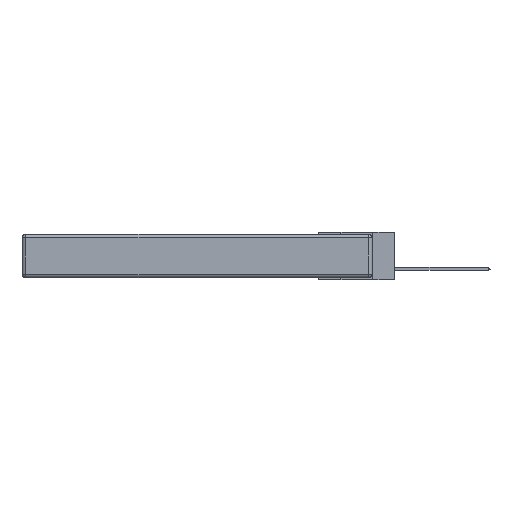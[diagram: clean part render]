
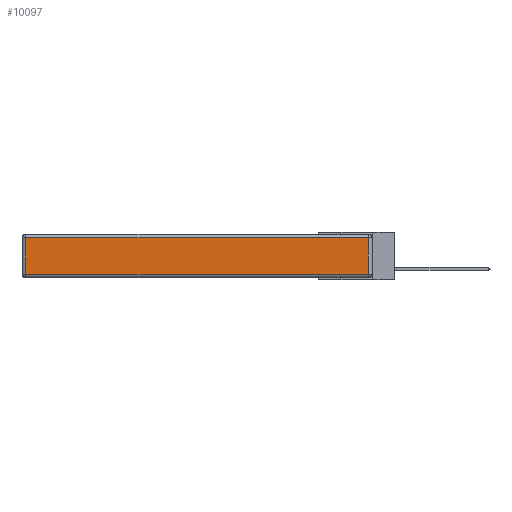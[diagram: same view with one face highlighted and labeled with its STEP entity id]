
A CAD part, left-side view. The second image highlights one B-rep face of the part: STEP entity #10097.
In plain terms, the highlighted planar face has unit normal (-1, 0, 0).
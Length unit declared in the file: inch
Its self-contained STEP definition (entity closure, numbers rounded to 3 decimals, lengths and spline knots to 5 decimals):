
#135 = PLANE ( 'NONE',  #2481 ) ;
#1014 = VERTEX_POINT ( 'NONE', #3017 ) ;
#1389 = DIRECTION ( 'NONE',  ( -1., 0., 0. ) ) ;
#1457 = VECTOR ( 'NONE', #16479, 39.37008 ) ;
#1952 = LINE ( 'NONE', #11635, #1457 ) ;
#2481 = AXIS2_PLACEMENT_3D ( 'NONE', #10940, #1389, #3572 ) ;
#2852 = LINE ( 'NONE', #8675, #4326 ) ;
#3017 = CARTESIAN_POINT ( 'NONE',  ( 0., 0.03, -0.313 ) ) ;
#3572 = DIRECTION ( 'NONE',  ( 0., 0., 1. ) ) ;
#4326 = VECTOR ( 'NONE', #10217, 39.37008 ) ;
#4814 = VERTEX_POINT ( 'NONE', #11718 ) ;
#5615 = DIRECTION ( 'NONE',  ( 0., 0., 1. ) ) ;
#6006 = ORIENTED_EDGE ( 'NONE', *, *, #6234, .T. ) ;
#6234 = EDGE_CURVE ( 'NONE', #6746, #4814, #2852, .T. ) ;
#6425 = EDGE_CURVE ( 'NONE', #4814, #11969, #17354, .T. ) ;
#6746 = VERTEX_POINT ( 'NONE', #12084 ) ;
#7591 = DIRECTION ( 'NONE',  ( 0., 0., -1. ) ) ;
#8225 = EDGE_LOOP ( 'NONE', ( #14822, #13582, #6006, #10631 ) ) ;
#8675 = CARTESIAN_POINT ( 'NONE',  ( 0., 2.75, -0.03 ) ) ;
#9130 = VECTOR ( 'NONE', #7591, 39.37008 ) ;
#9183 = VECTOR ( 'NONE', #5615, 39.37008 ) ;
#10097 = ADVANCED_FACE ( 'NONE', ( #10682 ), #135, .T. ) ;
#10148 = CARTESIAN_POINT ( 'NONE',  ( 0., 0.03, -0.343 ) ) ;
#10194 = EDGE_CURVE ( 'NONE', #11969, #1014, #1952, .T. ) ;
#10217 = DIRECTION ( 'NONE',  ( 0., 1., 0. ) ) ;
#10631 = ORIENTED_EDGE ( 'NONE', *, *, #6425, .T. ) ;
#10682 = FACE_OUTER_BOUND ( 'NONE', #8225, .T. ) ;
#10940 = CARTESIAN_POINT ( 'NONE',  ( 0., 0., -0.343 ) ) ;
#11520 = CARTESIAN_POINT ( 'NONE',  ( 0., 2.72, -0.313 ) ) ;
#11635 = CARTESIAN_POINT ( 'NONE',  ( 0., 0., -0.313 ) ) ;
#11718 = CARTESIAN_POINT ( 'NONE',  ( 0., 2.72, -0.03 ) ) ;
#11969 = VERTEX_POINT ( 'NONE', #11520 ) ;
#12084 = CARTESIAN_POINT ( 'NONE',  ( 0., 0.03, -0.03 ) ) ;
#12359 = CARTESIAN_POINT ( 'NONE',  ( 0., 2.72, -0.343 ) ) ;
#12822 = LINE ( 'NONE', #10148, #9183 ) ;
#13582 = ORIENTED_EDGE ( 'NONE', *, *, #18258, .T. ) ;
#14822 = ORIENTED_EDGE ( 'NONE', *, *, #10194, .T. ) ;
#16479 = DIRECTION ( 'NONE',  ( 0., -1., 0. ) ) ;
#17354 = LINE ( 'NONE', #12359, #9130 ) ;
#18258 = EDGE_CURVE ( 'NONE', #1014, #6746, #12822, .T. ) ;
